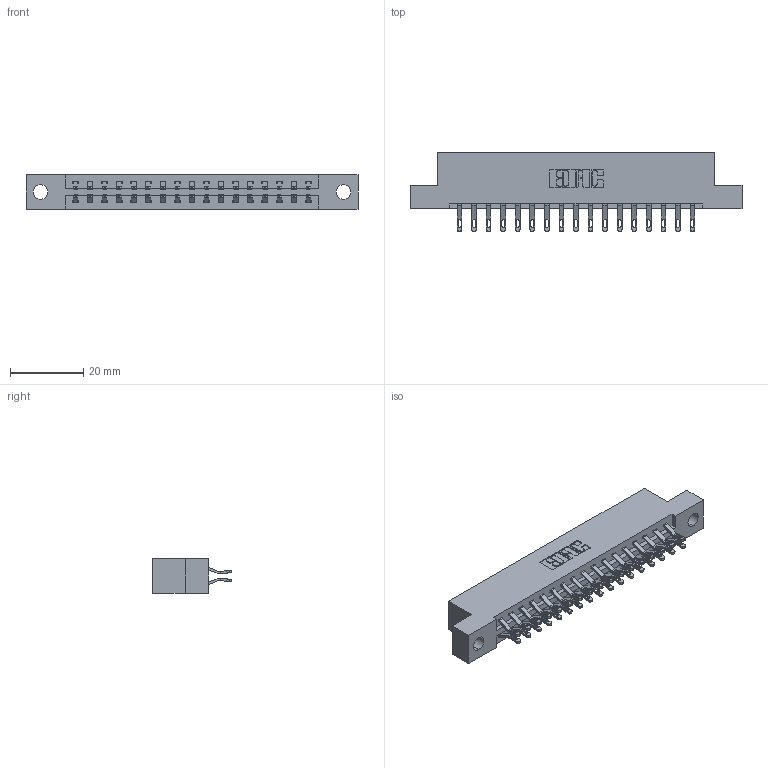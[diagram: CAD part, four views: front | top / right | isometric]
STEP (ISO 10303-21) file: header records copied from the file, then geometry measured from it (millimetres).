
FILE_DESCRIPTION (( 'STEP AP203' ), '1' );
FILE_NAME ('387-034-555-204.STEP', '2019-10-17T17:54:48', ( '' ), ( '' ), 'SwSTEP 2.0', 'SolidWorks 2016', '' );
FILE_SCHEMA (( 'CONFIG_CONTROL_DESIGN' ));
Length unit declared in the file: inch
Products named in the file (3): 345-292-001_555 Tail; 337 Part_Flush Mounting Lugs - 0.156 Dia-TH; 387-034-555-204
Assembly tree (35 placements, depth 2):
  387-034-555-204
    337 Part_Flush Mounting Lugs - 0.156 Dia-TH
    345-292-001_555 Tail  x34
Bounding box: 90.37 x 21.47 x 9.4 mm (x, y, z)
Volume: 9202.2 mm3; surface area: 10329.3 mm2
Topology: 35 solids, 35 shells, 2154 faces, 6737 edges, 4490 vertices
Faces by surface type: plane 1294, cylinder 860
Entity records: 16743 total; most frequent: CARTESIAN_POINT 2876, ORIENTED_EDGE 2782, DIRECTION 2463, EDGE_CURVE 1391, LINE 1243, VECTOR 1243, VERTEX_POINT 926, AXIS2_PLACEMENT_3D 610
